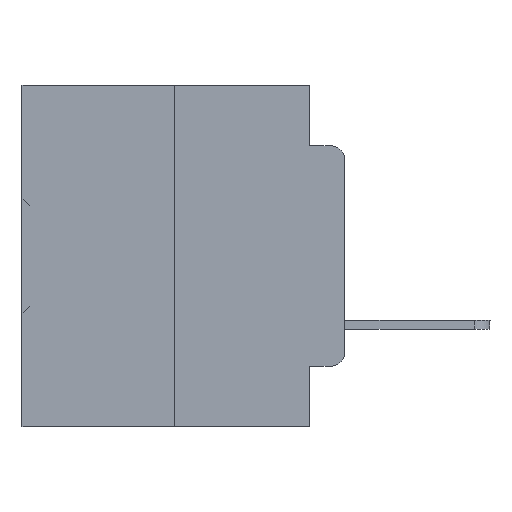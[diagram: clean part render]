
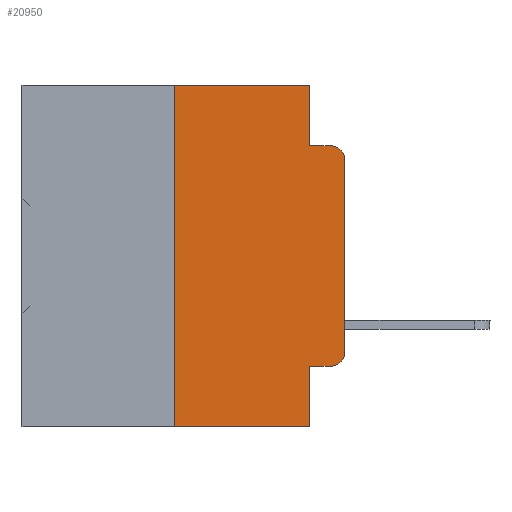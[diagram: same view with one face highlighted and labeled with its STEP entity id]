
A CAD part, left-side view. The second image highlights one B-rep face of the part: STEP entity #20950.
In plain terms, the highlighted planar face has unit normal (-1, 0, 0).
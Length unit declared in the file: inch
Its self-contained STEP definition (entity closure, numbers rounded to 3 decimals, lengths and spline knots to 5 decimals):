
#1123 = AXIS2_PLACEMENT_3D ( 'NONE', #8348, #8587, #20091 ) ;
#1740 = VERTEX_POINT ( 'NONE', #33023 ) ;
#2150 = EDGE_CURVE ( 'NONE', #20620, #14710, #6825, .T. ) ;
#2374 = VERTEX_POINT ( 'NONE', #25199 ) ;
#3218 = EDGE_CURVE ( 'NONE', #11191, #37300, #23450, .T. ) ;
#4352 = EDGE_CURVE ( 'NONE', #34588, #2374, #18814, .T. ) ;
#4923 = CARTESIAN_POINT ( 'NONE',  ( 0., 0.051, 0. ) ) ;
#5080 = LINE ( 'NONE', #25885, #14984 ) ;
#5100 = CARTESIAN_POINT ( 'NONE',  ( 0., 0.051, -0.0885 ) ) ;
#5508 = CARTESIAN_POINT ( 'NONE',  ( 0., 0.02, -0.0885 ) ) ;
#6108 = EDGE_CURVE ( 'NONE', #1740, #15214, #27024, .T. ) ;
#6228 = ORIENTED_EDGE ( 'NONE', *, *, #6108, .F. ) ;
#6825 = LINE ( 'NONE', #17347, #19902 ) ;
#7415 = PLANE ( 'NONE',  #35716 ) ;
#8348 = CARTESIAN_POINT ( 'NONE',  ( 0., 0.02, -0.1085 ) ) ;
#8449 = DIRECTION ( 'NONE',  ( 0., -1., 0. ) ) ;
#8456 = DIRECTION ( 'NONE',  ( 0., -1., 0. ) ) ;
#8584 = DIRECTION ( 'NONE',  ( 0., 0., -1. ) ) ;
#8587 = DIRECTION ( 'NONE',  ( -1., 0., 0. ) ) ;
#10120 = LINE ( 'NONE', #35091, #37207 ) ;
#10564 = ORIENTED_EDGE ( 'NONE', *, *, #18775, .T. ) ;
#10608 = DIRECTION ( 'NONE',  ( 0., 0., -1. ) ) ;
#10926 = ORIENTED_EDGE ( 'NONE', *, *, #10968, .T. ) ;
#10968 = EDGE_CURVE ( 'NONE', #1740, #23176, #33843, .T. ) ;
#11191 = VERTEX_POINT ( 'NONE', #5100 ) ;
#11572 = LINE ( 'NONE', #25029, #18382 ) ;
#12397 = FACE_OUTER_BOUND ( 'NONE', #32494, .T. ) ;
#13484 = CARTESIAN_POINT ( 'NONE',  ( 0., 0.051, -0.5 ) ) ;
#13811 = DIRECTION ( 'NONE',  ( 0., 0., -1. ) ) ;
#13892 = VECTOR ( 'NONE', #13811, 39.37008 ) ;
#14344 = CIRCLE ( 'NONE', #1123, 0.02 ) ;
#14710 = VERTEX_POINT ( 'NONE', #4923 ) ;
#14927 = ORIENTED_EDGE ( 'NONE', *, *, #30678, .T. ) ;
#14984 = VECTOR ( 'NONE', #8456, 39.37008 ) ;
#15214 = VERTEX_POINT ( 'NONE', #13484 ) ;
#15606 = CARTESIAN_POINT ( 'NONE',  ( 0., 0.473, 0. ) ) ;
#15864 = VERTEX_POINT ( 'NONE', #36640 ) ;
#16531 = ORIENTED_EDGE ( 'NONE', *, *, #21262, .F. ) ;
#17347 = CARTESIAN_POINT ( 'NONE',  ( 0., 0.473, 0. ) ) ;
#17401 = CARTESIAN_POINT ( 'NONE',  ( 0., 0.051, -0.0885 ) ) ;
#17492 = CIRCLE ( 'NONE', #25535, 0.02 ) ;
#18382 = VECTOR ( 'NONE', #10608, 39.37008 ) ;
#18775 = EDGE_CURVE ( 'NONE', #2374, #37300, #14344, .T. ) ;
#18814 = LINE ( 'NONE', #28403, #34121 ) ;
#18879 = DIRECTION ( 'NONE',  ( 0., -1., 0. ) ) ;
#18895 = DIRECTION ( 'NONE',  ( 1., 0., 0. ) ) ;
#19902 = VECTOR ( 'NONE', #23174, 39.37008 ) ;
#20091 = DIRECTION ( 'NONE',  ( 0., 0., -1. ) ) ;
#20620 = VERTEX_POINT ( 'NONE', #32126 ) ;
#20950 = ADVANCED_FACE ( 'NONE', ( #12397 ), #7415, .F. ) ;
#21029 = CARTESIAN_POINT ( 'NONE',  ( 0., 0.02, -0.4115 ) ) ;
#21262 = EDGE_CURVE ( 'NONE', #15864, #20620, #10120, .T. ) ;
#22721 = DIRECTION ( 'NONE',  ( 0., 0., 1. ) ) ;
#23174 = DIRECTION ( 'NONE',  ( 0., -1., 0. ) ) ;
#23176 = VERTEX_POINT ( 'NONE', #21029 ) ;
#23450 = LINE ( 'NONE', #17401, #32433 ) ;
#24008 = ORIENTED_EDGE ( 'NONE', *, *, #3218, .F. ) ;
#25029 = CARTESIAN_POINT ( 'NONE',  ( 0., 0.051, 0. ) ) ;
#25199 = CARTESIAN_POINT ( 'NONE',  ( 0., 0., -0.1085 ) ) ;
#25535 = AXIS2_PLACEMENT_3D ( 'NONE', #34921, #29304, #8584 ) ;
#25885 = CARTESIAN_POINT ( 'NONE',  ( 0., 0.473, -0.5 ) ) ;
#26800 = EDGE_CURVE ( 'NONE', #14710, #11191, #11572, .T. ) ;
#27024 = LINE ( 'NONE', #28202, #13892 ) ;
#27896 = ORIENTED_EDGE ( 'NONE', *, *, #26800, .F. ) ;
#28202 = CARTESIAN_POINT ( 'NONE',  ( 0., 0.051, 0. ) ) ;
#28403 = CARTESIAN_POINT ( 'NONE',  ( 0., 0., 0. ) ) ;
#29304 = DIRECTION ( 'NONE',  ( -1., 0., 0. ) ) ;
#29674 = ORIENTED_EDGE ( 'NONE', *, *, #33075, .T. ) ;
#30596 = CARTESIAN_POINT ( 'NONE',  ( 0., 0., -0.3915 ) ) ;
#30678 = EDGE_CURVE ( 'NONE', #15864, #15214, #5080, .T. ) ;
#32126 = CARTESIAN_POINT ( 'NONE',  ( 0., 0.25, 0. ) ) ;
#32433 = VECTOR ( 'NONE', #8449, 39.37008 ) ;
#32494 = EDGE_LOOP ( 'NONE', ( #33698, #10564, #24008, #27896, #34738, #16531, #14927, #6228, #10926, #29674 ) ) ;
#32951 = VECTOR ( 'NONE', #18879, 39.37008 ) ;
#33023 = CARTESIAN_POINT ( 'NONE',  ( 0., 0.051, -0.4115 ) ) ;
#33075 = EDGE_CURVE ( 'NONE', #23176, #34588, #17492, .T. ) ;
#33698 = ORIENTED_EDGE ( 'NONE', *, *, #4352, .T. ) ;
#33843 = LINE ( 'NONE', #36014, #32951 ) ;
#34121 = VECTOR ( 'NONE', #22721, 39.37008 ) ;
#34588 = VERTEX_POINT ( 'NONE', #30596 ) ;
#34738 = ORIENTED_EDGE ( 'NONE', *, *, #2150, .F. ) ;
#34823 = DIRECTION ( 'NONE',  ( 0., 0., 1. ) ) ;
#34921 = CARTESIAN_POINT ( 'NONE',  ( 0., 0.02, -0.3915 ) ) ;
#35091 = CARTESIAN_POINT ( 'NONE',  ( 0., 0.25, 0. ) ) ;
#35716 = AXIS2_PLACEMENT_3D ( 'NONE', #15606, #18895, #35773 ) ;
#35773 = DIRECTION ( 'NONE',  ( 0., 0., -1. ) ) ;
#36014 = CARTESIAN_POINT ( 'NONE',  ( 0., 0.051, -0.4115 ) ) ;
#36640 = CARTESIAN_POINT ( 'NONE',  ( 0., 0.25, -0.5 ) ) ;
#37207 = VECTOR ( 'NONE', #34823, 39.37008 ) ;
#37300 = VERTEX_POINT ( 'NONE', #5508 ) ;
